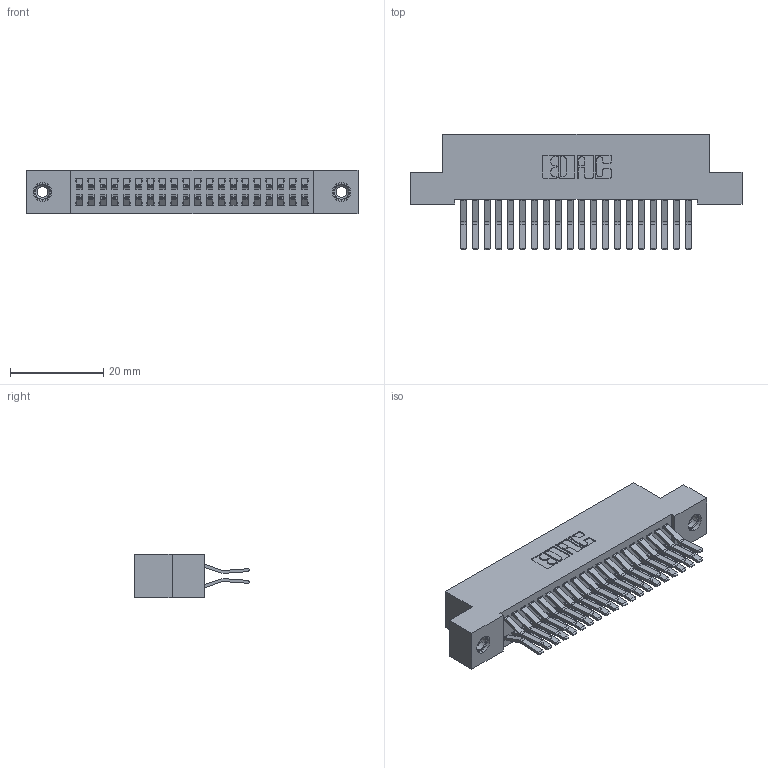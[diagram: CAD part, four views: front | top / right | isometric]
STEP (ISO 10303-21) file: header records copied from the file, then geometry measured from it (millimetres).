
FILE_DESCRIPTION (( 'STEP AP203' ), '1' );
FILE_NAME ('392-040-560-208.STEP', '2018-08-16T12:41:03', ( '' ), ( '' ), 'SwSTEP 2.0', 'SolidWorks 2016', '' );
FILE_SCHEMA (( 'CONFIG_CONTROL_DESIGN' ));
Length unit declared in the file: inch
Products named in the file (4): 342 Part_TI; 345-292-001_560 Tail; 345-250-001_345-250-003-102; 392-040-560-208
Assembly tree (43 placements, depth 2):
  392-040-560-208
    342 Part_TI
    345-292-001_560 Tail  x40
    345-250-001_345-250-003-102  x2
Bounding box: 71.12 x 24.78 x 9.4 mm (x, y, z)
Volume: 6542.9 mm3; surface area: 10748.1 mm2
Topology: 43 solids, 43 shells, 2330 faces, 6875 edges, 4522 vertices
Faces by surface type: plane 1538, cylinder 776, cone 12, torus 4
Entity records: 16854 total; most frequent: CARTESIAN_POINT 2801, ORIENTED_EDGE 2730, DIRECTION 2467, EDGE_CURVE 1365, VECTOR 1213, LINE 1213, VERTEX_POINT 904, AXIS2_PLACEMENT_3D 627
